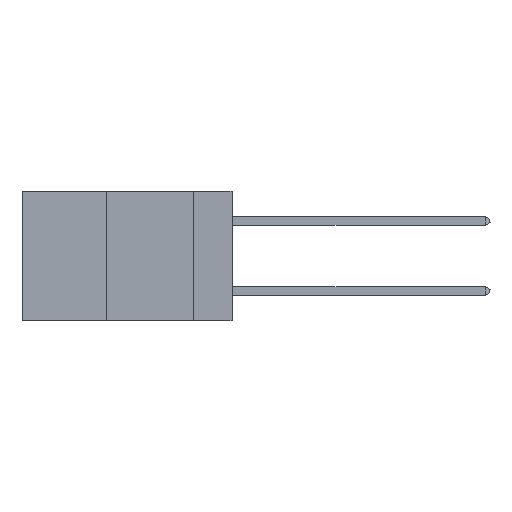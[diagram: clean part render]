
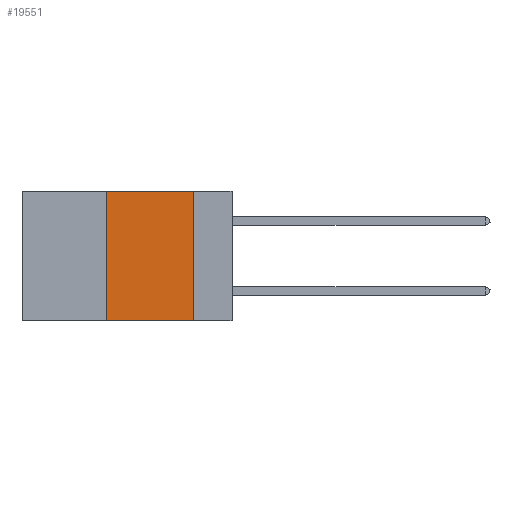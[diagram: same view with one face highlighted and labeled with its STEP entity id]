
A CAD part, left-side view. The second image highlights one B-rep face of the part: STEP entity #19551.
In plain terms, the highlighted planar face has unit normal (-1, 0, 0).
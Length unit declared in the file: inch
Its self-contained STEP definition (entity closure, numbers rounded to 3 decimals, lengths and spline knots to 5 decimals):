
#248 = ORIENTED_EDGE ( 'NONE', *, *, #24800, .F. ) ;
#1403 = PLANE ( 'NONE',  #10562 ) ;
#3098 = VERTEX_POINT ( 'NONE', #7117 ) ;
#5539 = CARTESIAN_POINT ( 'NONE',  ( 0., 0.6, 0. ) ) ;
#7117 = CARTESIAN_POINT ( 'NONE',  ( 0., 0.11, 0. ) ) ;
#7891 = VERTEX_POINT ( 'NONE', #13176 ) ;
#8001 = EDGE_CURVE ( 'NONE', #7891, #3098, #14119, .T. ) ;
#8322 = EDGE_CURVE ( 'NONE', #3098, #13375, #33520, .T. ) ;
#10096 = DIRECTION ( 'NONE',  ( 1., 0., 0. ) ) ;
#10562 = AXIS2_PLACEMENT_3D ( 'NONE', #27057, #10096, #29882 ) ;
#10661 = VECTOR ( 'NONE', #12950, 39.37008 ) ;
#12313 = CARTESIAN_POINT ( 'NONE',  ( 0., 0.11, -0.37 ) ) ;
#12950 = DIRECTION ( 'NONE',  ( 0., -1., 0. ) ) ;
#13176 = CARTESIAN_POINT ( 'NONE',  ( 0., 0.36, 0. ) ) ;
#13375 = VERTEX_POINT ( 'NONE', #12313 ) ;
#14051 = CARTESIAN_POINT ( 'NONE',  ( 0., 0.36, 0. ) ) ;
#14119 = LINE ( 'NONE', #5539, #28306 ) ;
#17339 = VERTEX_POINT ( 'NONE', #20346 ) ;
#17846 = EDGE_LOOP ( 'NONE', ( #29189, #26127, #248, #23056 ) ) ;
#19551 = ADVANCED_FACE ( 'NONE', ( #33169 ), #1403, .F. ) ;
#20346 = CARTESIAN_POINT ( 'NONE',  ( 0., 0.36, -0.37 ) ) ;
#20356 = LINE ( 'NONE', #14051, #28758 ) ;
#23056 = ORIENTED_EDGE ( 'NONE', *, *, #29743, .T. ) ;
#24800 = EDGE_CURVE ( 'NONE', #17339, #7891, #20356, .T. ) ;
#25729 = LINE ( 'NONE', #27191, #10661 ) ;
#26081 = VECTOR ( 'NONE', #29580, 39.37008 ) ;
#26127 = ORIENTED_EDGE ( 'NONE', *, *, #8001, .F. ) ;
#27057 = CARTESIAN_POINT ( 'NONE',  ( 0., 0.6, 0. ) ) ;
#27191 = CARTESIAN_POINT ( 'NONE',  ( 0., 0.6, -0.37 ) ) ;
#28306 = VECTOR ( 'NONE', #31085, 39.37008 ) ;
#28758 = VECTOR ( 'NONE', #33795, 39.37008 ) ;
#29189 = ORIENTED_EDGE ( 'NONE', *, *, #8322, .F. ) ;
#29580 = DIRECTION ( 'NONE',  ( 0., 0., -1. ) ) ;
#29743 = EDGE_CURVE ( 'NONE', #17339, #13375, #25729, .T. ) ;
#29882 = DIRECTION ( 'NONE',  ( 0., 0., -1. ) ) ;
#31085 = DIRECTION ( 'NONE',  ( 0., -1., 0. ) ) ;
#33169 = FACE_OUTER_BOUND ( 'NONE', #17846, .T. ) ;
#33520 = LINE ( 'NONE', #35057, #26081 ) ;
#33795 = DIRECTION ( 'NONE',  ( 0., 0., 1. ) ) ;
#35057 = CARTESIAN_POINT ( 'NONE',  ( 0., 0.11, 0. ) ) ;
